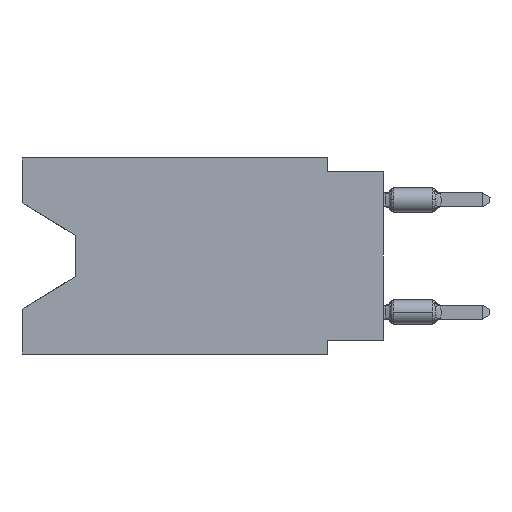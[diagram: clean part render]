
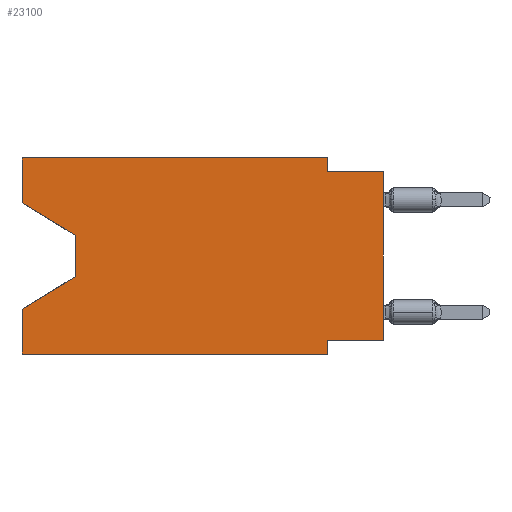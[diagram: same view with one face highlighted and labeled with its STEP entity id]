
A CAD part, left-side view. The second image highlights one B-rep face of the part: STEP entity #23100.
In plain terms, the highlighted planar face has unit normal (-1, 0, 0).
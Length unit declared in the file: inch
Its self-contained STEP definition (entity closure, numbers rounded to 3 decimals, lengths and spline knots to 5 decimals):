
#130 = CARTESIAN_POINT ( 'NONE',  ( 0., 0., -0.325 ) ) ;
#140 = CARTESIAN_POINT ( 'NONE',  ( 0., 0.1, -0.025 ) ) ;
#210 = DIRECTION ( 'NONE',  ( 0., 1., 0. ) ) ;
#370 = VERTEX_POINT ( 'NONE', #28570 ) ;
#637 = CARTESIAN_POINT ( 'NONE',  ( 0., 0., -0.025 ) ) ;
#808 = LINE ( 'NONE', #29171, #3363 ) ;
#1574 = VECTOR ( 'NONE', #10783, 39.37008 ) ;
#1989 = DIRECTION ( 'NONE',  ( 0., -1., 0. ) ) ;
#2618 = FACE_OUTER_BOUND ( 'NONE', #21356, .T. ) ;
#2729 = VECTOR ( 'NONE', #18129, 39.37008 ) ;
#2743 = VECTOR ( 'NONE', #210, 39.37008 ) ;
#2752 = CARTESIAN_POINT ( 'NONE',  ( 0., 0.645, 0. ) ) ;
#3005 = CARTESIAN_POINT ( 'NONE',  ( 0., 0.1, -0.35 ) ) ;
#3046 = CARTESIAN_POINT ( 'NONE',  ( 0., 0.645, 0. ) ) ;
#3287 = EDGE_CURVE ( 'NONE', #36071, #10375, #34592, .T. ) ;
#3363 = VECTOR ( 'NONE', #32184, 39.37008 ) ;
#4268 = VECTOR ( 'NONE', #14588, 39.37008 ) ;
#4962 = CARTESIAN_POINT ( 'NONE',  ( 0., 0., -0.025 ) ) ;
#5022 = VECTOR ( 'NONE', #18773, 39.37008 ) ;
#5101 = CARTESIAN_POINT ( 'NONE',  ( 0., 0.645, 0. ) ) ;
#6270 = LINE ( 'NONE', #3046, #4268 ) ;
#7147 = VECTOR ( 'NONE', #15194, 39.37008 ) ;
#7209 = CARTESIAN_POINT ( 'NONE',  ( 0., 0.645, -0.35 ) ) ;
#7614 = ORIENTED_EDGE ( 'NONE', *, *, #23264, .T. ) ;
#8221 = ORIENTED_EDGE ( 'NONE', *, *, #19330, .T. ) ;
#8308 = DIRECTION ( 'NONE',  ( 0., 0., -1. ) ) ;
#9695 = EDGE_CURVE ( 'NONE', #370, #21884, #12076, .T. ) ;
#10184 = VECTOR ( 'NONE', #16444, 39.37008 ) ;
#10375 = VERTEX_POINT ( 'NONE', #28397 ) ;
#10783 = DIRECTION ( 'NONE',  ( 0., 0., 1. ) ) ;
#12076 = LINE ( 'NONE', #29060, #27931 ) ;
#12171 = LINE ( 'NONE', #21048, #7147 ) ;
#12238 = CARTESIAN_POINT ( 'NONE',  ( 0., 0.1, 0. ) ) ;
#12905 = ORIENTED_EDGE ( 'NONE', *, *, #23298, .F. ) ;
#13311 = LINE ( 'NONE', #4962, #5022 ) ;
#13469 = DIRECTION ( 'NONE',  ( 0., -0.855, -0.519 ) ) ;
#13918 = VERTEX_POINT ( 'NONE', #12238 ) ;
#14346 = VERTEX_POINT ( 'NONE', #637 ) ;
#14411 = EDGE_CURVE ( 'NONE', #34105, #14346, #13311, .T. ) ;
#14588 = DIRECTION ( 'NONE',  ( 0., 0., 1. ) ) ;
#15194 = DIRECTION ( 'NONE',  ( 0., 0., 1. ) ) ;
#15201 = VECTOR ( 'NONE', #13469, 39.37008 ) ;
#15219 = EDGE_CURVE ( 'NONE', #27023, #13918, #16732, .T. ) ;
#15858 = CARTESIAN_POINT ( 'NONE',  ( 0., 0.55, -0.138 ) ) ;
#16307 = CARTESIAN_POINT ( 'NONE',  ( 0., 0.645, -0.08025 ) ) ;
#16444 = DIRECTION ( 'NONE',  ( 0., -1., 0. ) ) ;
#16732 = LINE ( 'NONE', #31081, #25539 ) ;
#17241 = EDGE_CURVE ( 'NONE', #34881, #21884, #33986, .T. ) ;
#17754 = PLANE ( 'NONE',  #27519 ) ;
#18129 = DIRECTION ( 'NONE',  ( 0., 0., -1. ) ) ;
#18290 = ORIENTED_EDGE ( 'NONE', *, *, #9695, .T. ) ;
#18623 = ORIENTED_EDGE ( 'NONE', *, *, #17241, .F. ) ;
#18773 = DIRECTION ( 'NONE',  ( 0., -1., 0. ) ) ;
#19096 = LINE ( 'NONE', #7209, #10184 ) ;
#19330 = EDGE_CURVE ( 'NONE', #34881, #24548, #19096, .T. ) ;
#21048 = CARTESIAN_POINT ( 'NONE',  ( 0., 0., 0. ) ) ;
#21356 = EDGE_LOOP ( 'NONE', ( #35280, #7614, #18290, #18623, #8221, #12905, #32616, #31567, #28924, #24196, #27328, #22965 ) ) ;
#21884 = VERTEX_POINT ( 'NONE', #27781 ) ;
#22965 = ORIENTED_EDGE ( 'NONE', *, *, #24126, .F. ) ;
#23100 = ADVANCED_FACE ( 'NONE', ( #2618 ), #17754, .F. ) ;
#23264 = EDGE_CURVE ( 'NONE', #25662, #370, #27198, .T. ) ;
#23298 = EDGE_CURVE ( 'NONE', #10375, #24548, #29653, .T. ) ;
#23470 = CARTESIAN_POINT ( 'NONE',  ( 0., 0., -0.325 ) ) ;
#23583 = EDGE_CURVE ( 'NONE', #13918, #34105, #808, .T. ) ;
#24126 = EDGE_CURVE ( 'NONE', #31783, #27023, #6270, .T. ) ;
#24196 = ORIENTED_EDGE ( 'NONE', *, *, #23583, .F. ) ;
#24548 = VERTEX_POINT ( 'NONE', #3005 ) ;
#25131 = EDGE_CURVE ( 'NONE', #31783, #25662, #27826, .T. ) ;
#25539 = VECTOR ( 'NONE', #1989, 39.37008 ) ;
#25662 = VERTEX_POINT ( 'NONE', #35047 ) ;
#27023 = VERTEX_POINT ( 'NONE', #2752 ) ;
#27198 = LINE ( 'NONE', #15858, #32305 ) ;
#27328 = ORIENTED_EDGE ( 'NONE', *, *, #15219, .F. ) ;
#27519 = AXIS2_PLACEMENT_3D ( 'NONE', #31728, #34167, #8308 ) ;
#27781 = CARTESIAN_POINT ( 'NONE',  ( 0., 0.645, -0.26975 ) ) ;
#27826 = LINE ( 'NONE', #16307, #15201 ) ;
#27931 = VECTOR ( 'NONE', #32265, 39.37008 ) ;
#28397 = CARTESIAN_POINT ( 'NONE',  ( 0., 0.1, -0.325 ) ) ;
#28570 = CARTESIAN_POINT ( 'NONE',  ( 0., 0.55, -0.212 ) ) ;
#28924 = ORIENTED_EDGE ( 'NONE', *, *, #14411, .F. ) ;
#29060 = CARTESIAN_POINT ( 'NONE',  ( 0., 0.55, -0.212 ) ) ;
#29171 = CARTESIAN_POINT ( 'NONE',  ( 0., 0.1, 0. ) ) ;
#29473 = DIRECTION ( 'NONE',  ( 0., 0., -1. ) ) ;
#29653 = LINE ( 'NONE', #35302, #2729 ) ;
#31081 = CARTESIAN_POINT ( 'NONE',  ( 0., 0.645, 0. ) ) ;
#31567 = ORIENTED_EDGE ( 'NONE', *, *, #35085, .T. ) ;
#31728 = CARTESIAN_POINT ( 'NONE',  ( 0., 0.645, 0. ) ) ;
#31783 = VERTEX_POINT ( 'NONE', #33752 ) ;
#32184 = DIRECTION ( 'NONE',  ( 0., 0., -1. ) ) ;
#32265 = DIRECTION ( 'NONE',  ( 0., 0.855, -0.519 ) ) ;
#32305 = VECTOR ( 'NONE', #29473, 39.37008 ) ;
#32616 = ORIENTED_EDGE ( 'NONE', *, *, #3287, .F. ) ;
#33752 = CARTESIAN_POINT ( 'NONE',  ( 0., 0.645, -0.08025 ) ) ;
#33986 = LINE ( 'NONE', #5101, #1574 ) ;
#34105 = VERTEX_POINT ( 'NONE', #140 ) ;
#34167 = DIRECTION ( 'NONE',  ( 1., 0., 0. ) ) ;
#34592 = LINE ( 'NONE', #23470, #2743 ) ;
#34881 = VERTEX_POINT ( 'NONE', #36341 ) ;
#35047 = CARTESIAN_POINT ( 'NONE',  ( 0., 0.55, -0.138 ) ) ;
#35085 = EDGE_CURVE ( 'NONE', #36071, #14346, #12171, .T. ) ;
#35280 = ORIENTED_EDGE ( 'NONE', *, *, #25131, .T. ) ;
#35302 = CARTESIAN_POINT ( 'NONE',  ( 0., 0.1, -0.35 ) ) ;
#36071 = VERTEX_POINT ( 'NONE', #130 ) ;
#36341 = CARTESIAN_POINT ( 'NONE',  ( 0., 0.645, -0.35 ) ) ;
